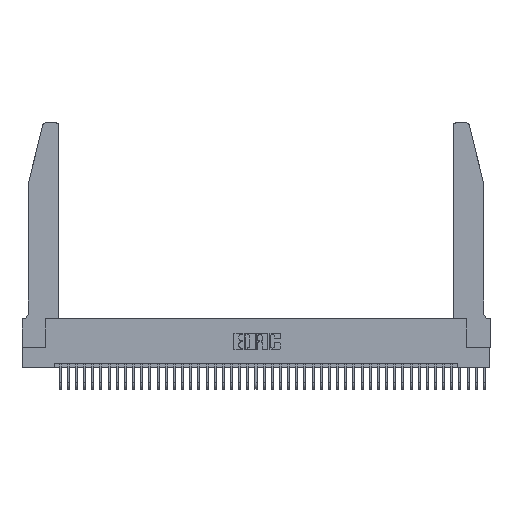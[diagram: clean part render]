
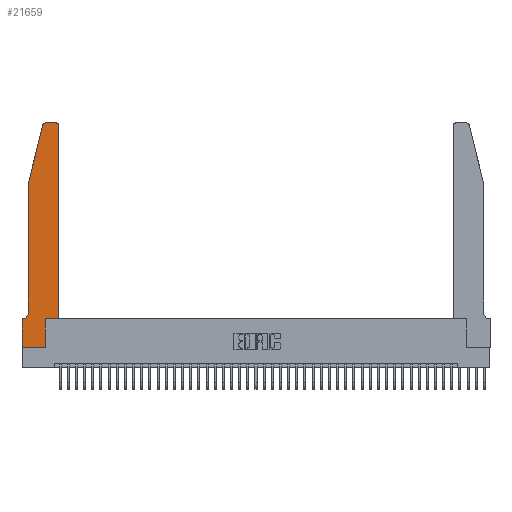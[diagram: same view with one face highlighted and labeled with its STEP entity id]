
A CAD part, top view. The second image highlights one B-rep face of the part: STEP entity #21659.
In plain terms, the highlighted planar face has unit normal (0, 0, 1).
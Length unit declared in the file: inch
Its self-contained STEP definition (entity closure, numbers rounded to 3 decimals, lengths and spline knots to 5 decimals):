
#121 = DIRECTION ( 'NONE',  ( 1., 0., 0. ) ) ;
#160 = LINE ( 'NONE', #20530, #16264 ) ;
#488 = EDGE_CURVE ( 'NONE', #38247, #39234, #5451, .T. ) ;
#669 = CARTESIAN_POINT ( 'NONE',  ( 0., 0., 0.37 ) ) ;
#1982 = EDGE_CURVE ( 'NONE', #23959, #26305, #12371, .T. ) ;
#2286 = ORIENTED_EDGE ( 'NONE', *, *, #11157, .T. ) ;
#2858 = CARTESIAN_POINT ( 'NONE',  ( 0.4505, 2.72, 0.37 ) ) ;
#3157 = EDGE_CURVE ( 'NONE', #28768, #23959, #160, .T. ) ;
#4933 = CARTESIAN_POINT ( 'NONE',  ( 0.0055, 0.42, 0.37 ) ) ;
#5451 = LINE ( 'NONE', #29740, #13027 ) ;
#5468 = CARTESIAN_POINT ( 'NONE',  ( 0.0055, 0.35, 0.37 ) ) ;
#6923 = VERTEX_POINT ( 'NONE', #5468 ) ;
#7431 = VECTOR ( 'NONE', #26177, 39.37008 ) ;
#7694 = EDGE_CURVE ( 'NONE', #6923, #28134, #39965, .T. ) ;
#8229 = DIRECTION ( 'NONE',  ( -1., 0., 0. ) ) ;
#8359 = VERTEX_POINT ( 'NONE', #29655 ) ;
#8457 = ORIENTED_EDGE ( 'NONE', *, *, #13126, .T. ) ;
#8579 = AXIS2_PLACEMENT_3D ( 'NONE', #17294, #39100, #20485 ) ;
#8780 = CARTESIAN_POINT ( 'NONE',  ( 0.4205, 2.72, 0.37 ) ) ;
#9247 = AXIS2_PLACEMENT_3D ( 'NONE', #12953, #19343, #121 ) ;
#10364 = CARTESIAN_POINT ( 'NONE',  ( 0.0755, 0.35, 0.37 ) ) ;
#11157 = EDGE_CURVE ( 'NONE', #33117, #38247, #23440, .T. ) ;
#11215 = EDGE_CURVE ( 'NONE', #34636, #6923, #26867, .T. ) ;
#11339 = CARTESIAN_POINT ( 'NONE',  ( 0.2865, 0.35, 0.37 ) ) ;
#11668 = EDGE_CURVE ( 'NONE', #19266, #8359, #32671, .T. ) ;
#11976 = DIRECTION ( 'NONE',  ( 1., 0., 0. ) ) ;
#12356 = DIRECTION ( 'NONE',  ( 0., -1., 0. ) ) ;
#12371 = LINE ( 'NONE', #28412, #22757 ) ;
#12953 = CARTESIAN_POINT ( 'NONE',  ( 0., 0.35, 0.37 ) ) ;
#13027 = VECTOR ( 'NONE', #32857, 39.37008 ) ;
#13126 = EDGE_CURVE ( 'NONE', #26305, #21517, #33977, .T. ) ;
#13185 = LINE ( 'NONE', #33817, #28992 ) ;
#13579 = DIRECTION ( 'NONE',  ( -1., 0., 0. ) ) ;
#14978 = EDGE_CURVE ( 'NONE', #39234, #34636, #13185, .T. ) ;
#15134 = EDGE_CURVE ( 'NONE', #28134, #19266, #33336, .T. ) ;
#15251 = CARTESIAN_POINT ( 'NONE',  ( 0.0755, 2., 0.37 ) ) ;
#15456 = CARTESIAN_POINT ( 'NONE',  ( 0.4205, 2.75, 0.37 ) ) ;
#15568 = CARTESIAN_POINT ( 'NONE',  ( 0., 0., 0.37 ) ) ;
#15872 = DIRECTION ( 'NONE',  ( 0., 1., 0. ) ) ;
#15899 = CARTESIAN_POINT ( 'NONE',  ( 0., 0., 0.37 ) ) ;
#16264 = VECTOR ( 'NONE', #17474, 39.37008 ) ;
#17294 = CARTESIAN_POINT ( 'NONE',  ( 0.284, 2.72, 0.37 ) ) ;
#17474 = DIRECTION ( 'NONE',  ( 1., 0., 0. ) ) ;
#18643 = ORIENTED_EDGE ( 'NONE', *, *, #24755, .T. ) ;
#19266 = VERTEX_POINT ( 'NONE', #15899 ) ;
#19343 = DIRECTION ( 'NONE',  ( 0., 0., 1. ) ) ;
#20349 = DIRECTION ( 'NONE',  ( -1., 0., 0. ) ) ;
#20485 = DIRECTION ( 'NONE',  ( 1., 0., 0. ) ) ;
#20530 = CARTESIAN_POINT ( 'NONE',  ( 0.4505, 0.35, 0.37 ) ) ;
#21098 = ORIENTED_EDGE ( 'NONE', *, *, #22550, .T. ) ;
#21358 = AXIS2_PLACEMENT_3D ( 'NONE', #4933, #27177, #8229 ) ;
#21517 = VERTEX_POINT ( 'NONE', #15456 ) ;
#21522 = ORIENTED_EDGE ( 'NONE', *, *, #3157, .T. ) ;
#21659 = ADVANCED_FACE ( 'NONE', ( #29016 ), #37986, .T. ) ;
#22550 = EDGE_CURVE ( 'NONE', #8359, #28768, #22691, .T. ) ;
#22691 = LINE ( 'NONE', #30911, #37298 ) ;
#22757 = VECTOR ( 'NONE', #15872, 39.37008 ) ;
#23440 = CIRCLE ( 'NONE', #8579, 0.03 ) ;
#23959 = VERTEX_POINT ( 'NONE', #25866 ) ;
#24755 = EDGE_CURVE ( 'NONE', #21517, #33117, #33349, .T. ) ;
#25094 = CARTESIAN_POINT ( 'NONE',  ( 0.0755, 0.42, 0.37 ) ) ;
#25866 = CARTESIAN_POINT ( 'NONE',  ( 0.4505, 0.35, 0.37 ) ) ;
#26177 = DIRECTION ( 'NONE',  ( 1., 0., 0. ) ) ;
#26305 = VERTEX_POINT ( 'NONE', #2858 ) ;
#26449 = EDGE_LOOP ( 'NONE', ( #18643, #2286, #40898, #35762, #32122, #31629, #29517, #36932, #21098, #21522, #26974, #8457 ) ) ;
#26867 = CIRCLE ( 'NONE', #21358, 0.07 ) ;
#26974 = ORIENTED_EDGE ( 'NONE', *, *, #1982, .T. ) ;
#26995 = VECTOR ( 'NONE', #12356, 39.37008 ) ;
#27003 = VECTOR ( 'NONE', #20349, 39.37008 ) ;
#27177 = DIRECTION ( 'NONE',  ( 0., 0., -1. ) ) ;
#28134 = VERTEX_POINT ( 'NONE', #39183 ) ;
#28412 = CARTESIAN_POINT ( 'NONE',  ( 0.4505, 0.35, 0.37 ) ) ;
#28768 = VERTEX_POINT ( 'NONE', #11339 ) ;
#28992 = VECTOR ( 'NONE', #36889, 39.37008 ) ;
#29016 = FACE_OUTER_BOUND ( 'NONE', #26449, .T. ) ;
#29517 = ORIENTED_EDGE ( 'NONE', *, *, #15134, .T. ) ;
#29655 = CARTESIAN_POINT ( 'NONE',  ( 0.2865, 0., 0.37 ) ) ;
#29740 = CARTESIAN_POINT ( 'NONE',  ( 0.0755, 2., 0.37 ) ) ;
#30062 = AXIS2_PLACEMENT_3D ( 'NONE', #8780, #30882, #11976 ) ;
#30882 = DIRECTION ( 'NONE',  ( 0., 0., 1. ) ) ;
#30911 = CARTESIAN_POINT ( 'NONE',  ( 0.2865, 0.35, 0.37 ) ) ;
#31629 = ORIENTED_EDGE ( 'NONE', *, *, #7694, .T. ) ;
#32122 = ORIENTED_EDGE ( 'NONE', *, *, #11215, .T. ) ;
#32671 = LINE ( 'NONE', #669, #7431 ) ;
#32857 = DIRECTION ( 'NONE',  ( -0.239, -0.971, 0. ) ) ;
#33117 = VERTEX_POINT ( 'NONE', #40282 ) ;
#33336 = LINE ( 'NONE', #15568, #26995 ) ;
#33349 = LINE ( 'NONE', #35845, #27003 ) ;
#33817 = CARTESIAN_POINT ( 'NONE',  ( 0.0755, 2., 0.37 ) ) ;
#33977 = CIRCLE ( 'NONE', #30062, 0.03 ) ;
#34636 = VERTEX_POINT ( 'NONE', #25094 ) ;
#35707 = CARTESIAN_POINT ( 'NONE',  ( 0.25487, 2.72718, 0.37 ) ) ;
#35762 = ORIENTED_EDGE ( 'NONE', *, *, #14978, .T. ) ;
#35845 = CARTESIAN_POINT ( 'NONE',  ( 0.2605, 2.75, 0.37 ) ) ;
#36889 = DIRECTION ( 'NONE',  ( 0., -1., 0. ) ) ;
#36932 = ORIENTED_EDGE ( 'NONE', *, *, #11668, .T. ) ;
#37103 = DIRECTION ( 'NONE',  ( 0., 1., 0. ) ) ;
#37298 = VECTOR ( 'NONE', #37103, 39.37008 ) ;
#37986 = PLANE ( 'NONE',  #9247 ) ;
#38247 = VERTEX_POINT ( 'NONE', #35707 ) ;
#38997 = VECTOR ( 'NONE', #13579, 39.37008 ) ;
#39100 = DIRECTION ( 'NONE',  ( 0., 0., 1. ) ) ;
#39183 = CARTESIAN_POINT ( 'NONE',  ( 0., 0.35, 0.37 ) ) ;
#39234 = VERTEX_POINT ( 'NONE', #15251 ) ;
#39965 = LINE ( 'NONE', #10364, #38997 ) ;
#40282 = CARTESIAN_POINT ( 'NONE',  ( 0.284, 2.75, 0.37 ) ) ;
#40898 = ORIENTED_EDGE ( 'NONE', *, *, #488, .T. ) ;
